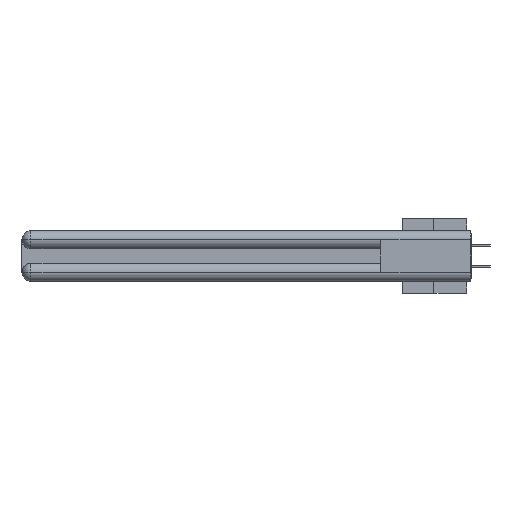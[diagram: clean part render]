
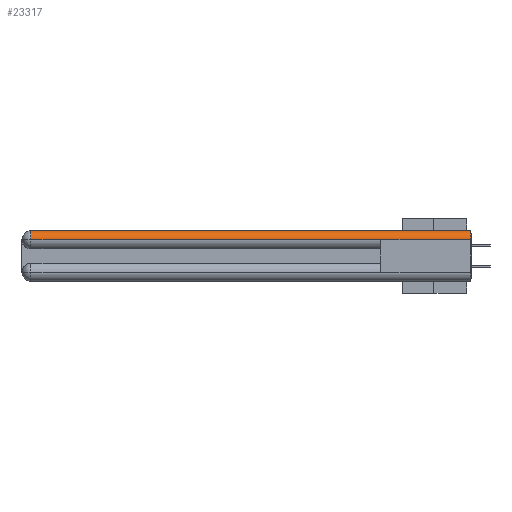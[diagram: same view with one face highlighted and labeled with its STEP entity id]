
A CAD part, left-side view. The second image highlights one B-rep face of the part: STEP entity #23317.
In plain terms, the highlighted cylindrical face has radius 1.562 mm (diameter 3.124 mm), a partial arc.
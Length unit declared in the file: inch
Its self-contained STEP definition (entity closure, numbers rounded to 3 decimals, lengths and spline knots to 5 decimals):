
#75 = CARTESIAN_POINT ( 'NONE',  ( 0.0615, 0., 0. ) ) ;
#1044 = ORIENTED_EDGE ( 'NONE', *, *, #39020, .F. ) ;
#2112 = VERTEX_POINT ( 'NONE', #29328 ) ;
#3841 = DIRECTION ( 'NONE',  ( 0., 1., 0. ) ) ;
#5328 = EDGE_CURVE ( 'NONE', #18550, #24936, #10936, .T. ) ;
#6201 = EDGE_LOOP ( 'NONE', ( #1044, #21776, #40436, #46020, #18273 ) ) ;
#6420 = CARTESIAN_POINT ( 'NONE',  ( 0., 0., -0.0615 ) ) ;
#6525 = VERTEX_POINT ( 'NONE', #43023 ) ;
#6865 = VECTOR ( 'NONE', #21598, 39.37008 ) ;
#10936 = LINE ( 'NONE', #32690, #19887 ) ;
#11387 = CARTESIAN_POINT ( 'NONE',  ( 0.0615, 0., -0.0615 ) ) ;
#12469 = LINE ( 'NONE', #75, #6865 ) ;
#13579 = DIRECTION ( 'NONE',  ( 0., -1., 0. ) ) ;
#13794 = VECTOR ( 'NONE', #44852, 39.37008 ) ;
#14151 = CARTESIAN_POINT ( 'NONE',  ( 0., 2.94, -0.0615 ) ) ;
#14444 = AXIS2_PLACEMENT_3D ( 'NONE', #15848, #13579, #41712 ) ;
#14974 = DIRECTION ( 'NONE',  ( 0., -1., 0. ) ) ;
#15848 = CARTESIAN_POINT ( 'NONE',  ( 0.0615, 2.94, -0.0615 ) ) ;
#17473 = EDGE_CURVE ( 'NONE', #31639, #24936, #19976, .T. ) ;
#18273 = ORIENTED_EDGE ( 'NONE', *, *, #42115, .F. ) ;
#18550 = VERTEX_POINT ( 'NONE', #6420 ) ;
#18922 = DIRECTION ( 'NONE',  ( 1., 0., 0. ) ) ;
#19887 = VECTOR ( 'NONE', #32379, 39.37008 ) ;
#19976 = LINE ( 'NONE', #31168, #13794 ) ;
#21598 = DIRECTION ( 'NONE',  ( 0., -1., 0. ) ) ;
#21776 = ORIENTED_EDGE ( 'NONE', *, *, #40928, .T. ) ;
#22843 = CIRCLE ( 'NONE', #32961, 0.0615 ) ;
#23317 = ADVANCED_FACE ( 'NONE', ( #36936 ), #27433, .T. ) ;
#24936 = VERTEX_POINT ( 'NONE', #45270 ) ;
#25196 = CARTESIAN_POINT ( 'NONE',  ( 0.0615, 0., -0.0615 ) ) ;
#25943 = DIRECTION ( 'NONE',  ( 0., 0., 1. ) ) ;
#27433 = CYLINDRICAL_SURFACE ( 'NONE', #34330, 0.0615 ) ;
#29328 = CARTESIAN_POINT ( 'NONE',  ( 0.0615, 0., 0. ) ) ;
#29664 = CIRCLE ( 'NONE', #14444, 0.0615 ) ;
#31168 = CARTESIAN_POINT ( 'NONE',  ( 0., 3., -0.0615 ) ) ;
#31639 = VERTEX_POINT ( 'NONE', #14151 ) ;
#32379 = DIRECTION ( 'NONE',  ( 0., 1., 0. ) ) ;
#32690 = CARTESIAN_POINT ( 'NONE',  ( 0., 3., -0.0615 ) ) ;
#32961 = AXIS2_PLACEMENT_3D ( 'NONE', #11387, #14974, #18922 ) ;
#34330 = AXIS2_PLACEMENT_3D ( 'NONE', #25196, #3841, #25943 ) ;
#36936 = FACE_OUTER_BOUND ( 'NONE', #6201, .T. ) ;
#39020 = EDGE_CURVE ( 'NONE', #6525, #2112, #12469, .T. ) ;
#40436 = ORIENTED_EDGE ( 'NONE', *, *, #17473, .T. ) ;
#40928 = EDGE_CURVE ( 'NONE', #6525, #31639, #29664, .T. ) ;
#41712 = DIRECTION ( 'NONE',  ( 0., 0., 1. ) ) ;
#42115 = EDGE_CURVE ( 'NONE', #2112, #18550, #22843, .T. ) ;
#43023 = CARTESIAN_POINT ( 'NONE',  ( 0.0615, 2.94, 0. ) ) ;
#44852 = DIRECTION ( 'NONE',  ( 0., -1., 0. ) ) ;
#45270 = CARTESIAN_POINT ( 'NONE',  ( 0., 0.6, -0.0615 ) ) ;
#46020 = ORIENTED_EDGE ( 'NONE', *, *, #5328, .F. ) ;
